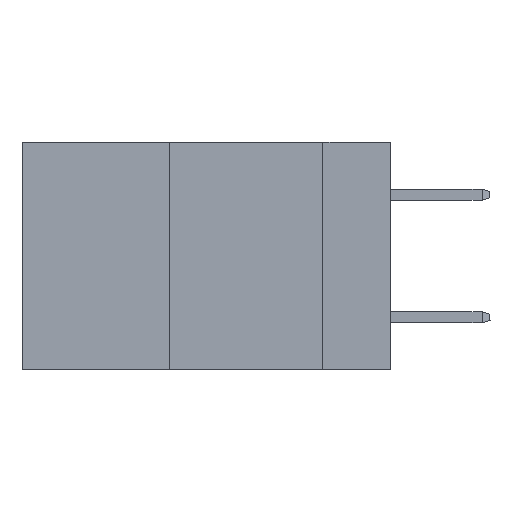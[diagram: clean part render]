
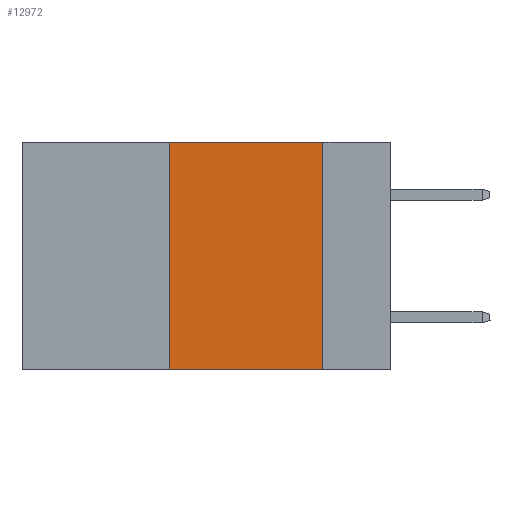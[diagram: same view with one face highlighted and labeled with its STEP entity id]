
A CAD part, left-side view. The second image highlights one B-rep face of the part: STEP entity #12972.
In plain terms, the highlighted planar face has unit normal (-1, 0, 0).
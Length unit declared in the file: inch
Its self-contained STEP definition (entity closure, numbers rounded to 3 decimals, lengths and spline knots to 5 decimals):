
#2294 = VERTEX_POINT ( 'NONE', #31592 ) ;
#2961 = CARTESIAN_POINT ( 'NONE',  ( 0., 0.36, 0. ) ) ;
#3122 = LINE ( 'NONE', #19256, #19742 ) ;
#4290 = ORIENTED_EDGE ( 'NONE', *, *, #23800, .F. ) ;
#6857 = LINE ( 'NONE', #22774, #15595 ) ;
#10725 = DIRECTION ( 'NONE',  ( 1., 0., 0. ) ) ;
#10930 = PLANE ( 'NONE',  #29502 ) ;
#12761 = DIRECTION ( 'NONE',  ( 0., 0., -1. ) ) ;
#12818 = VERTEX_POINT ( 'NONE', #38809 ) ;
#12972 = ADVANCED_FACE ( 'NONE', ( #14294 ), #10930, .F. ) ;
#14008 = EDGE_CURVE ( 'NONE', #12818, #35152, #14606, .T. ) ;
#14091 = CARTESIAN_POINT ( 'NONE',  ( 0., 0.6, 0. ) ) ;
#14294 = FACE_OUTER_BOUND ( 'NONE', #28155, .T. ) ;
#14606 = LINE ( 'NONE', #39970, #33585 ) ;
#15595 = VECTOR ( 'NONE', #35143, 39.37008 ) ;
#17110 = ORIENTED_EDGE ( 'NONE', *, *, #19823, .F. ) ;
#19256 = CARTESIAN_POINT ( 'NONE',  ( 0., 0.11, 0. ) ) ;
#19742 = VECTOR ( 'NONE', #12761, 39.37008 ) ;
#19823 = EDGE_CURVE ( 'NONE', #32057, #2294, #6857, .T. ) ;
#21713 = DIRECTION ( 'NONE',  ( 0., -1., 0. ) ) ;
#22774 = CARTESIAN_POINT ( 'NONE',  ( 0., 0.6, 0. ) ) ;
#23800 = EDGE_CURVE ( 'NONE', #12818, #32057, #28591, .T. ) ;
#24760 = ORIENTED_EDGE ( 'NONE', *, *, #14008, .T. ) ;
#27608 = ORIENTED_EDGE ( 'NONE', *, *, #37424, .F. ) ;
#28155 = EDGE_LOOP ( 'NONE', ( #27608, #17110, #4290, #24760 ) ) ;
#28187 = DIRECTION ( 'NONE',  ( 0., 0., 1. ) ) ;
#28591 = LINE ( 'NONE', #41162, #29192 ) ;
#29192 = VECTOR ( 'NONE', #28187, 39.37008 ) ;
#29502 = AXIS2_PLACEMENT_3D ( 'NONE', #14091, #10725, #33766 ) ;
#31592 = CARTESIAN_POINT ( 'NONE',  ( 0., 0.11, 0. ) ) ;
#32057 = VERTEX_POINT ( 'NONE', #2961 ) ;
#33585 = VECTOR ( 'NONE', #21713, 39.37008 ) ;
#33766 = DIRECTION ( 'NONE',  ( 0., 0., -1. ) ) ;
#35143 = DIRECTION ( 'NONE',  ( 0., -1., 0. ) ) ;
#35152 = VERTEX_POINT ( 'NONE', #39800 ) ;
#37424 = EDGE_CURVE ( 'NONE', #2294, #35152, #3122, .T. ) ;
#38809 = CARTESIAN_POINT ( 'NONE',  ( 0., 0.36, -0.37 ) ) ;
#39800 = CARTESIAN_POINT ( 'NONE',  ( 0., 0.11, -0.37 ) ) ;
#39970 = CARTESIAN_POINT ( 'NONE',  ( 0., 0.6, -0.37 ) ) ;
#41162 = CARTESIAN_POINT ( 'NONE',  ( 0., 0.36, 0. ) ) ;
